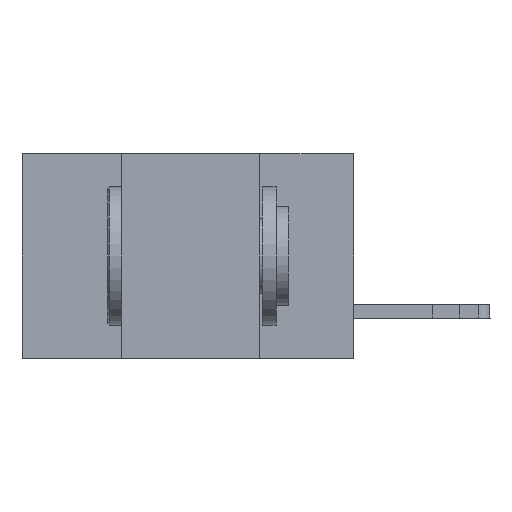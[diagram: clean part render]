
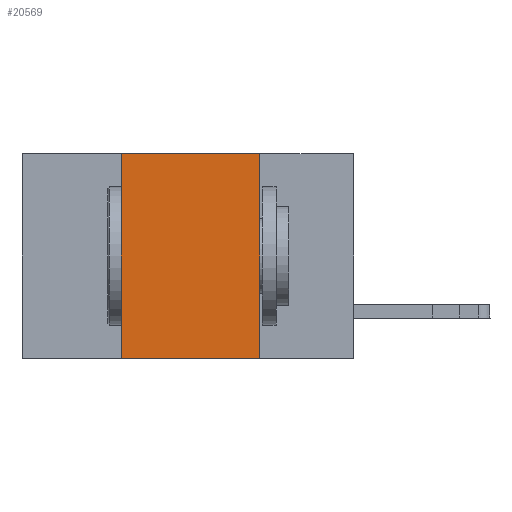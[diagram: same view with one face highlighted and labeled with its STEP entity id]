
A CAD part, left-side view. The second image highlights one B-rep face of the part: STEP entity #20569.
In plain terms, the highlighted planar face has unit normal (-1, 0, 0).
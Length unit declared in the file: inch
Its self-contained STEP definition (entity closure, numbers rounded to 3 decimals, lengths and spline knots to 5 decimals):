
#2473 = CARTESIAN_POINT ( 'NONE',  ( 0., 0.17, 0. ) ) ;
#3638 = VERTEX_POINT ( 'NONE', #26765 ) ;
#6310 = CARTESIAN_POINT ( 'NONE',  ( 0., 0.6, 0. ) ) ;
#6348 = LINE ( 'NONE', #9971, #27775 ) ;
#9465 = CARTESIAN_POINT ( 'NONE',  ( 0., 0.17, 0. ) ) ;
#9971 = CARTESIAN_POINT ( 'NONE',  ( 0., 0.6, -0.37 ) ) ;
#11410 = PLANE ( 'NONE',  #28720 ) ;
#12091 = EDGE_CURVE ( 'NONE', #19428, #16769, #13925, .T. ) ;
#12259 = EDGE_LOOP ( 'NONE', ( #23896, #22680, #30429, #17473 ) ) ;
#12430 = EDGE_CURVE ( 'NONE', #24521, #3638, #16601, .T. ) ;
#13086 = VECTOR ( 'NONE', #22280, 39.37008 ) ;
#13314 = EDGE_CURVE ( 'NONE', #16769, #24521, #26875, .T. ) ;
#13925 = LINE ( 'NONE', #21147, #13086 ) ;
#15698 = CARTESIAN_POINT ( 'NONE',  ( 0., 0.6, 0. ) ) ;
#16601 = LINE ( 'NONE', #2473, #21758 ) ;
#16769 = VERTEX_POINT ( 'NONE', #27132 ) ;
#17473 = ORIENTED_EDGE ( 'NONE', *, *, #20265, .T. ) ;
#17498 = CARTESIAN_POINT ( 'NONE',  ( 0., 0.42, -0.37 ) ) ;
#19428 = VERTEX_POINT ( 'NONE', #17498 ) ;
#19830 = DIRECTION ( 'NONE',  ( 1., 0., 0. ) ) ;
#20265 = EDGE_CURVE ( 'NONE', #19428, #3638, #6348, .T. ) ;
#20569 = ADVANCED_FACE ( 'NONE', ( #25639 ), #11410, .F. ) ;
#21147 = CARTESIAN_POINT ( 'NONE',  ( 0., 0.42, 0. ) ) ;
#21758 = VECTOR ( 'NONE', #22423, 39.37008 ) ;
#22280 = DIRECTION ( 'NONE',  ( 0., 0., 1. ) ) ;
#22423 = DIRECTION ( 'NONE',  ( 0., 0., -1. ) ) ;
#22680 = ORIENTED_EDGE ( 'NONE', *, *, #13314, .F. ) ;
#23896 = ORIENTED_EDGE ( 'NONE', *, *, #12430, .F. ) ;
#24521 = VERTEX_POINT ( 'NONE', #9465 ) ;
#25343 = DIRECTION ( 'NONE',  ( 0., 0., -1. ) ) ;
#25639 = FACE_OUTER_BOUND ( 'NONE', #12259, .T. ) ;
#26765 = CARTESIAN_POINT ( 'NONE',  ( 0., 0.17, -0.37 ) ) ;
#26875 = LINE ( 'NONE', #15698, #34958 ) ;
#27132 = CARTESIAN_POINT ( 'NONE',  ( 0., 0.42, 0. ) ) ;
#27775 = VECTOR ( 'NONE', #27787, 39.37008 ) ;
#27787 = DIRECTION ( 'NONE',  ( 0., -1., 0. ) ) ;
#28720 = AXIS2_PLACEMENT_3D ( 'NONE', #6310, #19830, #25343 ) ;
#30429 = ORIENTED_EDGE ( 'NONE', *, *, #12091, .F. ) ;
#32417 = DIRECTION ( 'NONE',  ( 0., -1., 0. ) ) ;
#34958 = VECTOR ( 'NONE', #32417, 39.37008 ) ;
